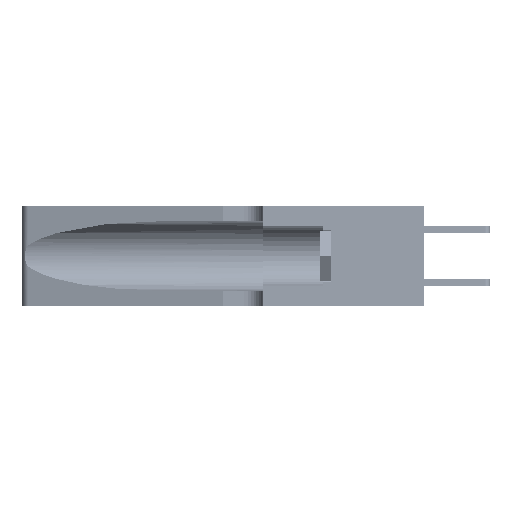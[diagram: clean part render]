
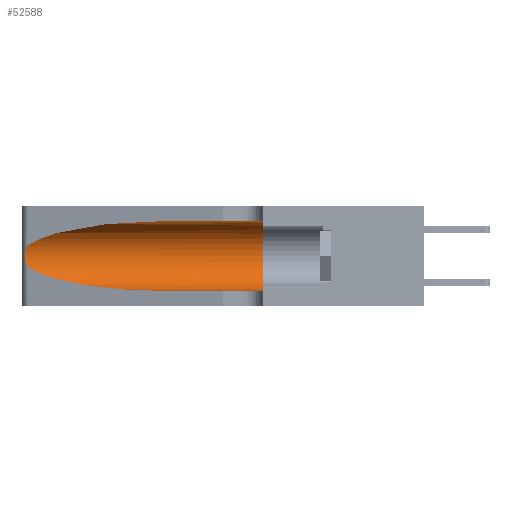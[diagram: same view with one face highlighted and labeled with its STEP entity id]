
A CAD part, left-side view. The second image highlights one B-rep face of the part: STEP entity #52588.
In plain terms, the highlighted cylindrical face has radius 3.308 mm (diameter 6.617 mm), a partial arc.
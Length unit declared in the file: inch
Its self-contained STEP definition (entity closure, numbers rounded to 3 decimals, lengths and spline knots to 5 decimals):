
#1447 = VERTEX_POINT ( 'NONE', #27752 ) ;
#1501 = CARTESIAN_POINT ( 'NONE',  ( 0.25639, 1.23186, 0.15144 ) ) ;
#4268 = EDGE_LOOP ( 'NONE', ( #22715, #48778, #52094, #27865, #54213, #11716 ) ) ;
#4647 = VERTEX_POINT ( 'NONE', #50186 ) ;
#5150 = VERTEX_POINT ( 'NONE', #8030 ) ;
#5692 =( BOUNDED_CURVE ( )  B_SPLINE_CURVE ( 3, ( #41325, #16137, #29061, #15045 ),
 .UNSPECIFIED., .F., .F. ) 
 B_SPLINE_CURVE_WITH_KNOTS ( ( 4, 4 ),
 ( 1.5708, 2.84003 ),
 .UNSPECIFIED. ) 
 CURVE ( )  GEOMETRIC_REPRESENTATION_ITEM ( )  RATIONAL_B_SPLINE_CURVE ( ( 1., 0.87, 0.87, 1. ) ) 
 REPRESENTATION_ITEM ( '' )  );
#5895 = VECTOR ( 'NONE', #37138, 39.37008 ) ;
#6127 = CARTESIAN_POINT ( 'NONE',  ( 0.25639, 1.23184, 0.21858 ) ) ;
#6629 = CARTESIAN_POINT ( 'NONE',  ( 0.1305, 1.61858, 0.185 ) ) ;
#8030 = CARTESIAN_POINT ( 'NONE',  ( 0.1305, 0.35, 0.05475 ) ) ;
#9062 =( BOUNDED_CURVE ( )  B_SPLINE_CURVE ( 3, ( #44266, #40753, #24456, #53691 ),
 .UNSPECIFIED., .F., .F. ) 
 B_SPLINE_CURVE_WITH_KNOTS ( ( 4, 4 ),
 ( 3.44316, 4.71239 ),
 .UNSPECIFIED. ) 
 CURVE ( )  GEOMETRIC_REPRESENTATION_ITEM ( )  RATIONAL_B_SPLINE_CURVE ( ( 1., 0.87, 0.87, 1. ) ) 
 REPRESENTATION_ITEM ( '' )  );
#9542 = AXIS2_PLACEMENT_3D ( 'NONE', #6629, #14729, #35534 ) ;
#10031 = CARTESIAN_POINT ( 'NONE',  ( 0.26075, 1.23896, 0.19203 ) ) ;
#10215 = CARTESIAN_POINT ( 'NONE',  ( 0.25555, 1.22994, 0.2215 ) ) ;
#10404 = CARTESIAN_POINT ( 'NONE',  ( 0.25856, 1.23593, 0.16098 ) ) ;
#11402 = CARTESIAN_POINT ( 'NONE',  ( 0.1305, 1.61858, 0.31525 ) ) ;
#11716 = ORIENTED_EDGE ( 'NONE', *, *, #36964, .F. ) ;
#13713 = CARTESIAN_POINT ( 'NONE',  ( 0.25487, 1.22718, 0.22369 ) ) ;
#14729 = DIRECTION ( 'NONE',  ( 0., -1., 0. ) ) ;
#15045 = CARTESIAN_POINT ( 'NONE',  ( 0.25487, 1.22718, 0.22369 ) ) ;
#16137 = CARTESIAN_POINT ( 'NONE',  ( 0.18966, 0.96281, 0.31525 ) ) ;
#18038 = CARTESIAN_POINT ( 'NONE',  ( 0.1305, 1.61858, 0.05475 ) ) ;
#18198 = VERTEX_POINT ( 'NONE', #40828 ) ;
#18661 = CARTESIAN_POINT ( 'NONE',  ( 0.25787, 1.23484, 0.2124 ) ) ;
#18699 = EDGE_CURVE ( 'NONE', #31459, #18198, #5692, .T. ) ;
#18848 = CARTESIAN_POINT ( 'NONE',  ( 0.25487, 1.22718, 0.14631 ) ) ;
#21023 = LINE ( 'NONE', #18038, #22999 ) ;
#22225 = VERTEX_POINT ( 'NONE', #45756 ) ;
#22715 = ORIENTED_EDGE ( 'NONE', *, *, #18699, .T. ) ;
#22981 = DIRECTION ( 'NONE',  ( 0., 0., 1. ) ) ;
#22999 = VECTOR ( 'NONE', #52087, 39.37008 ) ;
#23687 = LINE ( 'NONE', #11402, #5895 ) ;
#24456 = CARTESIAN_POINT ( 'NONE',  ( 0.18966, 0.96281, 0.05475 ) ) ;
#24622 = B_SPLINE_CURVE_WITH_KNOTS ( 'NONE', 3,
 ( #13713, #10215, #6127, #18661, #39262, #51809, #10031, #52540, #43311, #10404, #52160, #1501, #26630, #18848 ),
 .UNSPECIFIED., .F., .F.,
 ( 4, 2, 2, 2, 2, 2, 4 ),
 ( 0., 0.00027, 0.00053, 0.00107, 0.0016, 0.00187, 0.00214 ),
 .UNSPECIFIED. ) ;
#26630 = CARTESIAN_POINT ( 'NONE',  ( 0.25555, 1.22993, 0.14849 ) ) ;
#27752 = CARTESIAN_POINT ( 'NONE',  ( 0.25487, 1.22718, 0.14631 ) ) ;
#27865 = ORIENTED_EDGE ( 'NONE', *, *, #47339, .T. ) ;
#29061 = CARTESIAN_POINT ( 'NONE',  ( 0.2373, 1.15595, 0.28018 ) ) ;
#31459 = VERTEX_POINT ( 'NONE', #41366 ) ;
#34176 = FACE_OUTER_BOUND ( 'NONE', #4268, .T. ) ;
#35534 = DIRECTION ( 'NONE',  ( 0., 0., -1. ) ) ;
#36964 = EDGE_CURVE ( 'NONE', #31459, #4647, #23687, .T. ) ;
#37138 = DIRECTION ( 'NONE',  ( 0., -1., 0. ) ) ;
#37187 = AXIS2_PLACEMENT_3D ( 'NONE', #44238, #47779, #22981 ) ;
#39262 = CARTESIAN_POINT ( 'NONE',  ( 0.25854, 1.2359, 0.20912 ) ) ;
#40753 = CARTESIAN_POINT ( 'NONE',  ( 0.2373, 1.15595, 0.08982 ) ) ;
#40828 = CARTESIAN_POINT ( 'NONE',  ( 0.25487, 1.22718, 0.22369 ) ) ;
#41325 = CARTESIAN_POINT ( 'NONE',  ( 0.1305, 0.72297, 0.31525 ) ) ;
#41366 = CARTESIAN_POINT ( 'NONE',  ( 0.1305, 0.72297, 0.31525 ) ) ;
#41705 = CIRCLE ( 'NONE', #37187, 0.13025 ) ;
#43311 = CARTESIAN_POINT ( 'NONE',  ( 0.26017, 1.23833, 0.17102 ) ) ;
#44238 = CARTESIAN_POINT ( 'NONE',  ( 0.1305, 0.35, 0.185 ) ) ;
#44266 = CARTESIAN_POINT ( 'NONE',  ( 0.25487, 1.22718, 0.14631 ) ) ;
#45072 = EDGE_CURVE ( 'NONE', #4647, #5150, #41705, .T. ) ;
#45756 = CARTESIAN_POINT ( 'NONE',  ( 0.1305, 0.72297, 0.05475 ) ) ;
#46687 = CYLINDRICAL_SURFACE ( 'NONE', #9542, 0.13025 ) ;
#47339 = EDGE_CURVE ( 'NONE', #22225, #5150, #21023, .T. ) ;
#47779 = DIRECTION ( 'NONE',  ( 0., 1., 0. ) ) ;
#48558 = EDGE_CURVE ( 'NONE', #18198, #1447, #24622, .T. ) ;
#48778 = ORIENTED_EDGE ( 'NONE', *, *, #48558, .T. ) ;
#50186 = CARTESIAN_POINT ( 'NONE',  ( 0.1305, 0.35, 0.31525 ) ) ;
#51809 = CARTESIAN_POINT ( 'NONE',  ( 0.26018, 1.23835, 0.19895 ) ) ;
#52087 = DIRECTION ( 'NONE',  ( 0., -1., 0. ) ) ;
#52094 = ORIENTED_EDGE ( 'NONE', *, *, #53337, .T. ) ;
#52160 = CARTESIAN_POINT ( 'NONE',  ( 0.25789, 1.23486, 0.15765 ) ) ;
#52540 = CARTESIAN_POINT ( 'NONE',  ( 0.26075, 1.23896, 0.178 ) ) ;
#52588 = ADVANCED_FACE ( 'NONE', ( #34176 ), #46687, .F. ) ;
#53337 = EDGE_CURVE ( 'NONE', #1447, #22225, #9062, .T. ) ;
#53691 = CARTESIAN_POINT ( 'NONE',  ( 0.1305, 0.72297, 0.05475 ) ) ;
#54213 = ORIENTED_EDGE ( 'NONE', *, *, #45072, .F. ) ;
